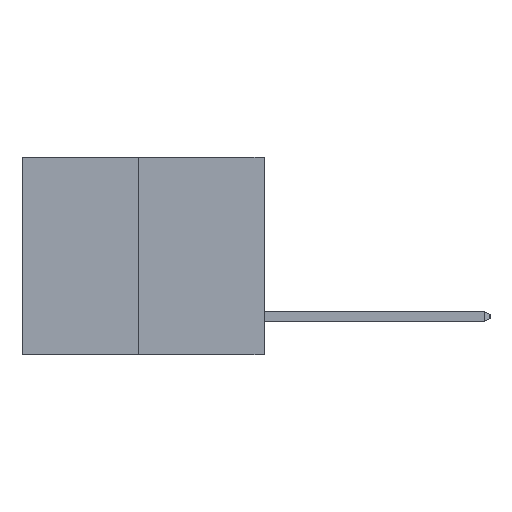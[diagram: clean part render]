
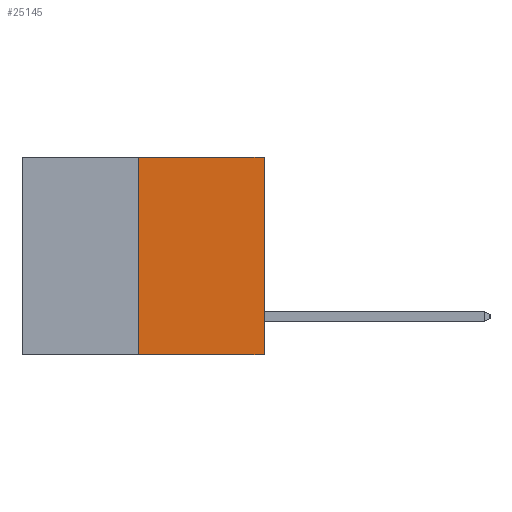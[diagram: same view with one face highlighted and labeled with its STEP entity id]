
A CAD part, left-side view. The second image highlights one B-rep face of the part: STEP entity #25145.
In plain terms, the highlighted planar face has unit normal (-1, 0, 0).
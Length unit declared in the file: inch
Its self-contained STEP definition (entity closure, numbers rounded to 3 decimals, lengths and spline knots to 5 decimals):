
#555 = LINE ( 'NONE', #5065, #21135 ) ;
#1730 = CARTESIAN_POINT ( 'NONE',  ( 0., 0.6, 0. ) ) ;
#1787 = CARTESIAN_POINT ( 'NONE',  ( 0., 0.6, -0.49 ) ) ;
#2382 = EDGE_CURVE ( 'NONE', #8400, #9304, #555, .T. ) ;
#4313 = VERTEX_POINT ( 'NONE', #19920 ) ;
#4619 = CARTESIAN_POINT ( 'NONE',  ( 0., 0.312, -0.49 ) ) ;
#5065 = CARTESIAN_POINT ( 'NONE',  ( 0., 0., 0. ) ) ;
#7144 = FACE_OUTER_BOUND ( 'NONE', #7930, .T. ) ;
#7930 = EDGE_LOOP ( 'NONE', ( #14517, #8112, #11149, #24545 ) ) ;
#8112 = ORIENTED_EDGE ( 'NONE', *, *, #16935, .T. ) ;
#8400 = VERTEX_POINT ( 'NONE', #18977 ) ;
#9267 = DIRECTION ( 'NONE',  ( 0., 0., 1. ) ) ;
#9304 = VERTEX_POINT ( 'NONE', #12253 ) ;
#9365 = VECTOR ( 'NONE', #9267, 39.37008 ) ;
#10007 = EDGE_CURVE ( 'NONE', #16660, #4313, #10926, .T. ) ;
#10035 = AXIS2_PLACEMENT_3D ( 'NONE', #16590, #12504, #20470 ) ;
#10926 = LINE ( 'NONE', #4619, #9365 ) ;
#11149 = ORIENTED_EDGE ( 'NONE', *, *, #2382, .T. ) ;
#12253 = CARTESIAN_POINT ( 'NONE',  ( 0., 0., 0. ) ) ;
#12318 = VECTOR ( 'NONE', #19291, 39.37008 ) ;
#12504 = DIRECTION ( 'NONE',  ( 1., 0., 0. ) ) ;
#12757 = PLANE ( 'NONE',  #10035 ) ;
#14517 = ORIENTED_EDGE ( 'NONE', *, *, #10007, .F. ) ;
#16590 = CARTESIAN_POINT ( 'NONE',  ( 0., 0.6, 0. ) ) ;
#16660 = VERTEX_POINT ( 'NONE', #25431 ) ;
#16935 = EDGE_CURVE ( 'NONE', #16660, #8400, #17197, .T. ) ;
#17010 = DIRECTION ( 'NONE',  ( 0., -1., 0. ) ) ;
#17197 = LINE ( 'NONE', #1787, #12318 ) ;
#18042 = LINE ( 'NONE', #1730, #23917 ) ;
#18829 = DIRECTION ( 'NONE',  ( 0., 0., 1. ) ) ;
#18977 = CARTESIAN_POINT ( 'NONE',  ( 0., 0., -0.49 ) ) ;
#19291 = DIRECTION ( 'NONE',  ( 0., -1., 0. ) ) ;
#19920 = CARTESIAN_POINT ( 'NONE',  ( 0., 0.312, 0. ) ) ;
#20470 = DIRECTION ( 'NONE',  ( 0., 0., -1. ) ) ;
#21135 = VECTOR ( 'NONE', #18829, 39.37008 ) ;
#23121 = EDGE_CURVE ( 'NONE', #4313, #9304, #18042, .T. ) ;
#23917 = VECTOR ( 'NONE', #17010, 39.37008 ) ;
#24545 = ORIENTED_EDGE ( 'NONE', *, *, #23121, .F. ) ;
#25145 = ADVANCED_FACE ( 'NONE', ( #7144 ), #12757, .F. ) ;
#25431 = CARTESIAN_POINT ( 'NONE',  ( 0., 0.312, -0.49 ) ) ;
